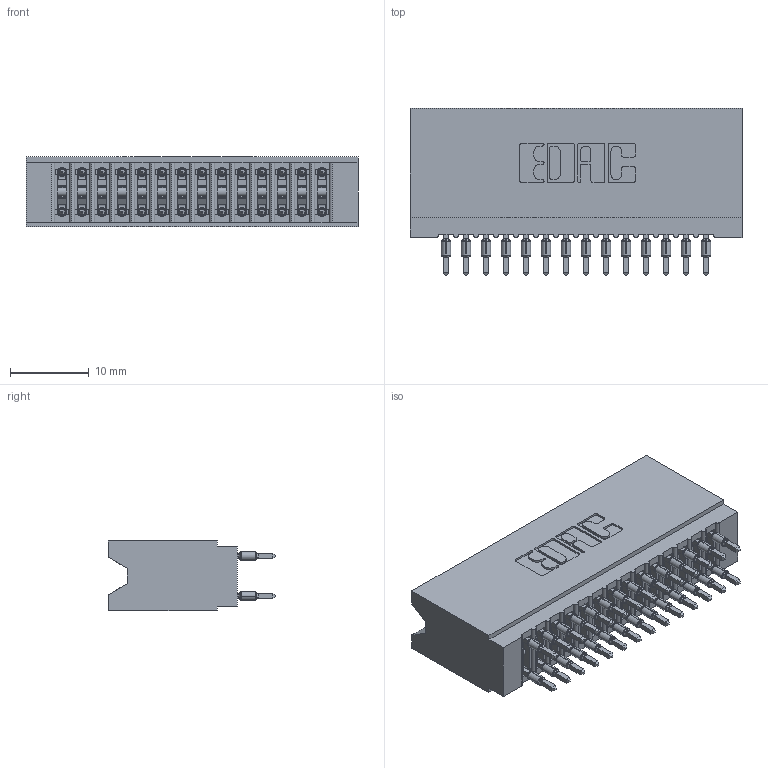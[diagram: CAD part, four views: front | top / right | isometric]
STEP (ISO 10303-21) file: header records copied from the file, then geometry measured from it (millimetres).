
FILE_DESCRIPTION (( 'STEP AP203' ), '1' );
FILE_NAME ('745-028-560-206.STEP', '2026-02-26T16:51:26', ( '' ), ( '' ), 'SwSTEP 2.0', 'SolidWorks 2023', '' );
FILE_SCHEMA (( 'CONFIG_CONTROL_DESIGN' ));
Length unit declared in the file: millimetre
Products named in the file (3): 745-292-001_560; 745-028-560-206; 745 Part_Insulator Option - 06
Assembly tree (29 placements, depth 2):
  745-028-560-206
    745 Part_Insulator Option - 06
    745-292-001_560  x28
Bounding box: 42.16 x 21.22 x 8.89 mm (x, y, z)
Volume: 4047.5 mm3; surface area: 8048.9 mm2
Topology: 29 solids, 29 shells, 2854 faces, 7806 edges, 4960 vertices
Faces by surface type: plane 1484, cylinder 642, bspline 560, torus 168
Entity records: 27735 total; most frequent: CARTESIAN_POINT 5324, ORIENTED_EDGE 4704, DIRECTION 4138, EDGE_CURVE 2352, VECTOR 2078, LINE 2078, VERTEX_POINT 1504, AXIS2_PLACEMENT_3D 1030
